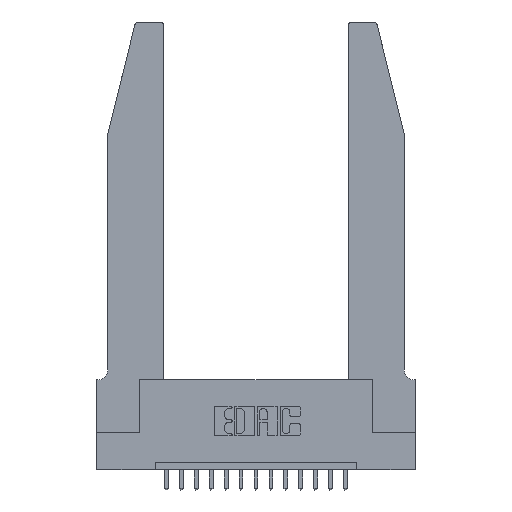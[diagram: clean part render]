
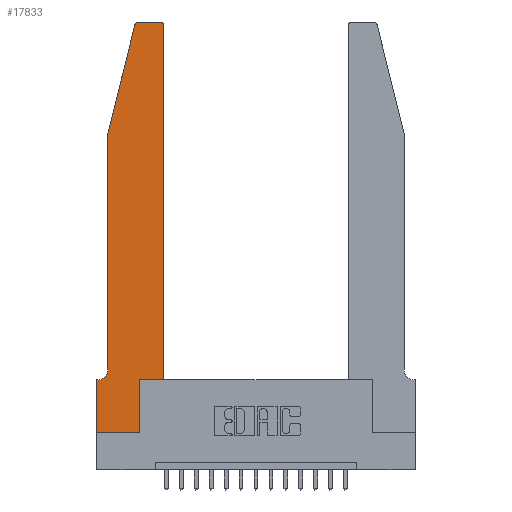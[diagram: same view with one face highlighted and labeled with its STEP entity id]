
A CAD part, top view. The second image highlights one B-rep face of the part: STEP entity #17833.
In plain terms, the highlighted planar face has unit normal (0, 0, 1).
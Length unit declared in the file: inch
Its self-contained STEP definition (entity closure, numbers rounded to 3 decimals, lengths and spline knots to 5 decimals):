
#325 = CARTESIAN_POINT ( 'NONE',  ( 0.4505, 2.72, 0.37 ) ) ;
#504 = ORIENTED_EDGE ( 'NONE', *, *, #10811, .T. ) ;
#729 = DIRECTION ( 'NONE',  ( 1., 0., 0. ) ) ;
#808 = EDGE_CURVE ( 'NONE', #6840, #11776, #14224, .T. ) ;
#1048 = LINE ( 'NONE', #3988, #9121 ) ;
#1104 = VERTEX_POINT ( 'NONE', #17221 ) ;
#1195 = VERTEX_POINT ( 'NONE', #14977 ) ;
#1243 = VECTOR ( 'NONE', #5699, 39.37008 ) ;
#1600 = LINE ( 'NONE', #16300, #12560 ) ;
#1720 = CARTESIAN_POINT ( 'NONE',  ( 0., 0., 0.37 ) ) ;
#2820 = CARTESIAN_POINT ( 'NONE',  ( 0.0755, 2., 0.37 ) ) ;
#3134 = CARTESIAN_POINT ( 'NONE',  ( 0.2865, 0.35, 0.37 ) ) ;
#3346 = VECTOR ( 'NONE', #11707, 39.37008 ) ;
#3505 = LINE ( 'NONE', #14545, #7104 ) ;
#3619 = VECTOR ( 'NONE', #14144, 39.37008 ) ;
#3709 = EDGE_CURVE ( 'NONE', #5617, #12327, #6543, .T. ) ;
#3751 = DIRECTION ( 'NONE',  ( 0., -1., 0. ) ) ;
#3782 = VERTEX_POINT ( 'NONE', #2820 ) ;
#3896 = ORIENTED_EDGE ( 'NONE', *, *, #10587, .T. ) ;
#3988 = CARTESIAN_POINT ( 'NONE',  ( 0., 0., 0.37 ) ) ;
#4177 = ORIENTED_EDGE ( 'NONE', *, *, #18426, .T. ) ;
#4205 = CARTESIAN_POINT ( 'NONE',  ( 0.0055, 0.42, 0.37 ) ) ;
#4436 = CARTESIAN_POINT ( 'NONE',  ( 0., 0.35, 0.37 ) ) ;
#4614 = CARTESIAN_POINT ( 'NONE',  ( 0.4205, 2.75, 0.37 ) ) ;
#4863 = CARTESIAN_POINT ( 'NONE',  ( 0.0755, 0.42, 0.37 ) ) ;
#5020 = VERTEX_POINT ( 'NONE', #4614 ) ;
#5358 = ORIENTED_EDGE ( 'NONE', *, *, #16337, .T. ) ;
#5389 = ORIENTED_EDGE ( 'NONE', *, *, #12222, .T. ) ;
#5442 = LINE ( 'NONE', #13172, #1243 ) ;
#5617 = VERTEX_POINT ( 'NONE', #4863 ) ;
#5699 = DIRECTION ( 'NONE',  ( -0.239, -0.971, 0. ) ) ;
#5965 = ORIENTED_EDGE ( 'NONE', *, *, #12642, .T. ) ;
#6090 = VECTOR ( 'NONE', #8786, 39.37008 ) ;
#6377 = CIRCLE ( 'NONE', #14849, 0.03 ) ;
#6543 = CIRCLE ( 'NONE', #10956, 0.07 ) ;
#6718 = AXIS2_PLACEMENT_3D ( 'NONE', #4436, #13200, #15871 ) ;
#6840 = VERTEX_POINT ( 'NONE', #13972 ) ;
#6920 = ORIENTED_EDGE ( 'NONE', *, *, #15033, .T. ) ;
#7104 = VECTOR ( 'NONE', #16164, 39.37008 ) ;
#7388 = PLANE ( 'NONE',  #6718 ) ;
#7687 = LINE ( 'NONE', #14847, #6090 ) ;
#7800 = CARTESIAN_POINT ( 'NONE',  ( 0.284, 2.72, 0.37 ) ) ;
#7962 = EDGE_CURVE ( 'NONE', #1195, #14871, #1048, .T. ) ;
#8255 = CARTESIAN_POINT ( 'NONE',  ( 0.2605, 2.75, 0.37 ) ) ;
#8261 = CARTESIAN_POINT ( 'NONE',  ( 0.2865, 0.35, 0.37 ) ) ;
#8786 = DIRECTION ( 'NONE',  ( 1., 0., 0. ) ) ;
#9121 = VECTOR ( 'NONE', #18109, 39.37008 ) ;
#9227 = DIRECTION ( 'NONE',  ( 1., 0., 0. ) ) ;
#9306 = FACE_OUTER_BOUND ( 'NONE', #12068, .T. ) ;
#9528 = CARTESIAN_POINT ( 'NONE',  ( 0.2865, 0., 0.37 ) ) ;
#9725 = DIRECTION ( 'NONE',  ( 0., 1., 0. ) ) ;
#10475 = VECTOR ( 'NONE', #3751, 39.37008 ) ;
#10587 = EDGE_CURVE ( 'NONE', #1104, #1195, #18315, .T. ) ;
#10811 = EDGE_CURVE ( 'NONE', #12327, #1104, #1600, .T. ) ;
#10933 = ORIENTED_EDGE ( 'NONE', *, *, #7962, .T. ) ;
#10956 = AXIS2_PLACEMENT_3D ( 'NONE', #4205, #14403, #11363 ) ;
#11045 = VECTOR ( 'NONE', #9725, 39.37008 ) ;
#11357 = DIRECTION ( 'NONE',  ( -1., 0., 0. ) ) ;
#11363 = DIRECTION ( 'NONE',  ( -1., 0., 0. ) ) ;
#11393 = ORIENTED_EDGE ( 'NONE', *, *, #11895, .T. ) ;
#11707 = DIRECTION ( 'NONE',  ( 0., -1., 0. ) ) ;
#11776 = VERTEX_POINT ( 'NONE', #16137 ) ;
#11844 = CARTESIAN_POINT ( 'NONE',  ( 0.0055, 0.35, 0.37 ) ) ;
#11895 = EDGE_CURVE ( 'NONE', #12913, #14522, #7687, .T. ) ;
#12068 = EDGE_LOOP ( 'NONE', ( #5389, #15442, #16217, #6920, #12959, #504, #3896, #10933, #5965, #11393, #4177, #5358 ) ) ;
#12222 = EDGE_CURVE ( 'NONE', #5020, #6840, #17049, .T. ) ;
#12327 = VERTEX_POINT ( 'NONE', #11844 ) ;
#12560 = VECTOR ( 'NONE', #11357, 39.37008 ) ;
#12642 = EDGE_CURVE ( 'NONE', #14871, #12913, #17035, .T. ) ;
#12913 = VERTEX_POINT ( 'NONE', #3134 ) ;
#12959 = ORIENTED_EDGE ( 'NONE', *, *, #3709, .T. ) ;
#13172 = CARTESIAN_POINT ( 'NONE',  ( 0.0755, 2., 0.37 ) ) ;
#13200 = DIRECTION ( 'NONE',  ( 0., 0., 1. ) ) ;
#13972 = CARTESIAN_POINT ( 'NONE',  ( 0.284, 2.75, 0.37 ) ) ;
#14144 = DIRECTION ( 'NONE',  ( -1., 0., 0. ) ) ;
#14207 = CARTESIAN_POINT ( 'NONE',  ( 0.4505, 0.35, 0.37 ) ) ;
#14224 = CIRCLE ( 'NONE', #16138, 0.03 ) ;
#14403 = DIRECTION ( 'NONE',  ( 0., 0., -1. ) ) ;
#14522 = VERTEX_POINT ( 'NONE', #14207 ) ;
#14545 = CARTESIAN_POINT ( 'NONE',  ( 0.4505, 0.35, 0.37 ) ) ;
#14847 = CARTESIAN_POINT ( 'NONE',  ( 0.4505, 0.35, 0.37 ) ) ;
#14849 = AXIS2_PLACEMENT_3D ( 'NONE', #16510, #14877, #9227 ) ;
#14871 = VERTEX_POINT ( 'NONE', #9528 ) ;
#14877 = DIRECTION ( 'NONE',  ( 0., 0., 1. ) ) ;
#14897 = DIRECTION ( 'NONE',  ( 0., 0., 1. ) ) ;
#14977 = CARTESIAN_POINT ( 'NONE',  ( 0., 0., 0.37 ) ) ;
#15033 = EDGE_CURVE ( 'NONE', #3782, #5617, #15364, .T. ) ;
#15312 = CARTESIAN_POINT ( 'NONE',  ( 0.0755, 2., 0.37 ) ) ;
#15364 = LINE ( 'NONE', #15312, #10475 ) ;
#15442 = ORIENTED_EDGE ( 'NONE', *, *, #808, .T. ) ;
#15871 = DIRECTION ( 'NONE',  ( 1., 0., 0. ) ) ;
#16137 = CARTESIAN_POINT ( 'NONE',  ( 0.25487, 2.72718, 0.37 ) ) ;
#16138 = AXIS2_PLACEMENT_3D ( 'NONE', #7800, #14897, #729 ) ;
#16164 = DIRECTION ( 'NONE',  ( 0., 1., 0. ) ) ;
#16217 = ORIENTED_EDGE ( 'NONE', *, *, #16749, .T. ) ;
#16230 = VERTEX_POINT ( 'NONE', #325 ) ;
#16300 = CARTESIAN_POINT ( 'NONE',  ( 0.0755, 0.35, 0.37 ) ) ;
#16337 = EDGE_CURVE ( 'NONE', #16230, #5020, #6377, .T. ) ;
#16510 = CARTESIAN_POINT ( 'NONE',  ( 0.4205, 2.72, 0.37 ) ) ;
#16749 = EDGE_CURVE ( 'NONE', #11776, #3782, #5442, .T. ) ;
#17035 = LINE ( 'NONE', #8261, #11045 ) ;
#17049 = LINE ( 'NONE', #8255, #3619 ) ;
#17221 = CARTESIAN_POINT ( 'NONE',  ( 0., 0.35, 0.37 ) ) ;
#17833 = ADVANCED_FACE ( 'NONE', ( #9306 ), #7388, .T. ) ;
#18109 = DIRECTION ( 'NONE',  ( 1., 0., 0. ) ) ;
#18315 = LINE ( 'NONE', #1720, #3346 ) ;
#18426 = EDGE_CURVE ( 'NONE', #14522, #16230, #3505, .T. ) ;
